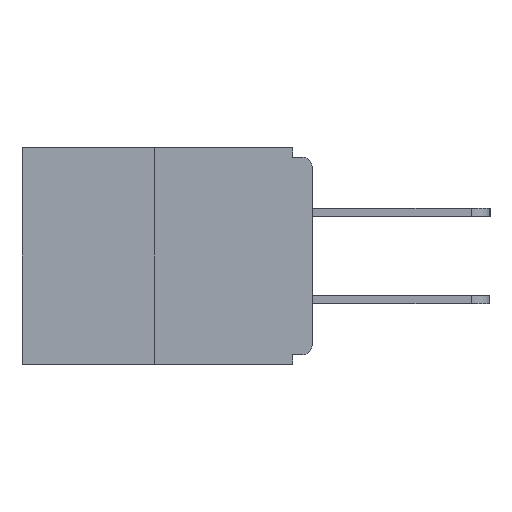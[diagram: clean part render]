
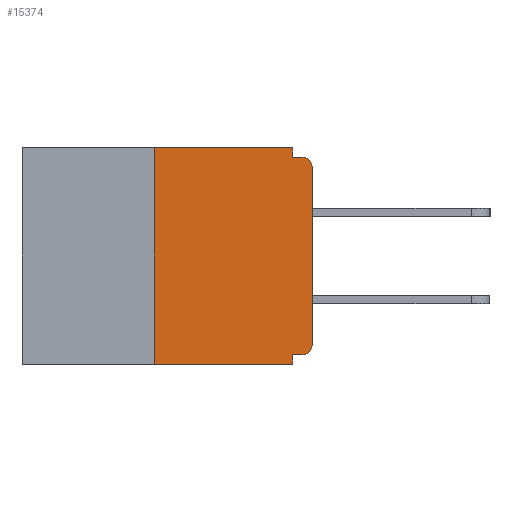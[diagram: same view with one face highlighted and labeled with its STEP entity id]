
A CAD part, left-side view. The second image highlights one B-rep face of the part: STEP entity #15374.
In plain terms, the highlighted planar face has unit normal (-1, 0, 0).
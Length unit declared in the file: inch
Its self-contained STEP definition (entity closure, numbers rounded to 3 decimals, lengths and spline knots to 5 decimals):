
#116 = ORIENTED_EDGE ( 'NONE', *, *, #5797, .F. ) ;
#548 = AXIS2_PLACEMENT_3D ( 'NONE', #4685, #12397, #15321 ) ;
#725 = VERTEX_POINT ( 'NONE', #12813 ) ;
#826 = ORIENTED_EDGE ( 'NONE', *, *, #8485, .T. ) ;
#909 = VECTOR ( 'NONE', #10721, 39.37008 ) ;
#1243 = EDGE_CURVE ( 'NONE', #17369, #4859, #12869, .T. ) ;
#1270 = DIRECTION ( 'NONE',  ( 0., 0., 1. ) ) ;
#1637 = LINE ( 'NONE', #8175, #12702 ) ;
#1675 = ORIENTED_EDGE ( 'NONE', *, *, #10460, .F. ) ;
#1790 = CIRCLE ( 'NONE', #548, 0.015 ) ;
#2052 = EDGE_CURVE ( 'NONE', #7994, #5197, #8822, .T. ) ;
#2444 = DIRECTION ( 'NONE',  ( 0., 0., -1. ) ) ;
#2753 = EDGE_CURVE ( 'NONE', #4544, #6234, #12340, .T. ) ;
#2941 = DIRECTION ( 'NONE',  ( 0., 1., 0. ) ) ;
#2968 = CARTESIAN_POINT ( 'NONE',  ( 0., 0.46, -0.343 ) ) ;
#3226 = VECTOR ( 'NONE', #10887, 39.37008 ) ;
#3380 = EDGE_CURVE ( 'NONE', #6234, #16784, #4997, .T. ) ;
#4280 = ORIENTED_EDGE ( 'NONE', *, *, #11982, .F. ) ;
#4544 = VERTEX_POINT ( 'NONE', #17344 ) ;
#4685 = CARTESIAN_POINT ( 'NONE',  ( 0., 0.015, -0.313 ) ) ;
#4764 = ORIENTED_EDGE ( 'NONE', *, *, #7035, .F. ) ;
#4859 = VERTEX_POINT ( 'NONE', #5698 ) ;
#4997 = CIRCLE ( 'NONE', #11948, 0.015 ) ;
#5197 = VERTEX_POINT ( 'NONE', #12374 ) ;
#5629 = EDGE_CURVE ( 'NONE', #18832, #5197, #1637, .T. ) ;
#5698 = CARTESIAN_POINT ( 'NONE',  ( 0., 0.031, -0.015 ) ) ;
#5797 = EDGE_CURVE ( 'NONE', #725, #17369, #9848, .T. ) ;
#6234 = VERTEX_POINT ( 'NONE', #7542 ) ;
#6397 = CARTESIAN_POINT ( 'NONE',  ( 0., 0.015, -0.03 ) ) ;
#7035 = EDGE_CURVE ( 'NONE', #7994, #725, #15952, .T. ) ;
#7080 = LINE ( 'NONE', #16276, #18006 ) ;
#7542 = CARTESIAN_POINT ( 'NONE',  ( 0., 0., -0.03 ) ) ;
#7641 = VECTOR ( 'NONE', #10596, 39.37008 ) ;
#7994 = VERTEX_POINT ( 'NONE', #11070 ) ;
#8175 = CARTESIAN_POINT ( 'NONE',  ( 0., 0.031, -0.343 ) ) ;
#8190 = EDGE_LOOP ( 'NONE', ( #116, #4764, #17671, #8336, #1675, #826, #17437, #17087, #4280, #19450 ) ) ;
#8336 = ORIENTED_EDGE ( 'NONE', *, *, #5629, .F. ) ;
#8485 = EDGE_CURVE ( 'NONE', #15748, #4544, #1790, .T. ) ;
#8822 = LINE ( 'NONE', #2968, #7641 ) ;
#9034 = VECTOR ( 'NONE', #15304, 39.37008 ) ;
#9529 = CARTESIAN_POINT ( 'NONE',  ( 0., 0.031, 0. ) ) ;
#9639 = CARTESIAN_POINT ( 'NONE',  ( 0., 0.015, -0.328 ) ) ;
#9848 = LINE ( 'NONE', #10450, #909 ) ;
#10426 = CARTESIAN_POINT ( 'NONE',  ( 0., 0., -0.328 ) ) ;
#10450 = CARTESIAN_POINT ( 'NONE',  ( 0., 0.46, 0. ) ) ;
#10460 = EDGE_CURVE ( 'NONE', #15748, #18832, #16341, .T. ) ;
#10596 = DIRECTION ( 'NONE',  ( 0., -1., 0. ) ) ;
#10721 = DIRECTION ( 'NONE',  ( 0., -1., 0. ) ) ;
#10887 = DIRECTION ( 'NONE',  ( 0., 0., -1. ) ) ;
#11070 = CARTESIAN_POINT ( 'NONE',  ( 0., 0.25, -0.343 ) ) ;
#11948 = AXIS2_PLACEMENT_3D ( 'NONE', #6397, #18716, #12524 ) ;
#11982 = EDGE_CURVE ( 'NONE', #4859, #16784, #7080, .T. ) ;
#12021 = DIRECTION ( 'NONE',  ( 0., -1., 0. ) ) ;
#12305 = DIRECTION ( 'NONE',  ( 1., 0., 0. ) ) ;
#12340 = LINE ( 'NONE', #18499, #9034 ) ;
#12374 = CARTESIAN_POINT ( 'NONE',  ( 0., 0.031, -0.343 ) ) ;
#12397 = DIRECTION ( 'NONE',  ( -1., 0., 0. ) ) ;
#12412 = CARTESIAN_POINT ( 'NONE',  ( 0., 0.031, 0. ) ) ;
#12524 = DIRECTION ( 'NONE',  ( 0., 0., -1. ) ) ;
#12702 = VECTOR ( 'NONE', #2444, 39.37008 ) ;
#12813 = CARTESIAN_POINT ( 'NONE',  ( 0., 0.25, 0. ) ) ;
#12869 = LINE ( 'NONE', #9529, #3226 ) ;
#13877 = CARTESIAN_POINT ( 'NONE',  ( 0., 0.031, -0.328 ) ) ;
#15304 = DIRECTION ( 'NONE',  ( 0., 0., 1. ) ) ;
#15321 = DIRECTION ( 'NONE',  ( 0., 0., -1. ) ) ;
#15374 = ADVANCED_FACE ( 'NONE', ( #17642 ), #16702, .F. ) ;
#15748 = VERTEX_POINT ( 'NONE', #9639 ) ;
#15952 = LINE ( 'NONE', #16166, #16171 ) ;
#16166 = CARTESIAN_POINT ( 'NONE',  ( 0., 0.25, 0. ) ) ;
#16171 = VECTOR ( 'NONE', #1270, 39.37008 ) ;
#16276 = CARTESIAN_POINT ( 'NONE',  ( 0., 0., -0.015 ) ) ;
#16341 = LINE ( 'NONE', #10426, #17104 ) ;
#16702 = PLANE ( 'NONE',  #17232 ) ;
#16784 = VERTEX_POINT ( 'NONE', #18428 ) ;
#16907 = CARTESIAN_POINT ( 'NONE',  ( 0., 0.46, 0. ) ) ;
#17087 = ORIENTED_EDGE ( 'NONE', *, *, #3380, .T. ) ;
#17104 = VECTOR ( 'NONE', #2941, 39.37008 ) ;
#17232 = AXIS2_PLACEMENT_3D ( 'NONE', #16907, #12305, #18367 ) ;
#17344 = CARTESIAN_POINT ( 'NONE',  ( 0., 0., -0.313 ) ) ;
#17369 = VERTEX_POINT ( 'NONE', #12412 ) ;
#17437 = ORIENTED_EDGE ( 'NONE', *, *, #2753, .T. ) ;
#17642 = FACE_OUTER_BOUND ( 'NONE', #8190, .T. ) ;
#17671 = ORIENTED_EDGE ( 'NONE', *, *, #2052, .T. ) ;
#18006 = VECTOR ( 'NONE', #12021, 39.37008 ) ;
#18367 = DIRECTION ( 'NONE',  ( 0., 0., -1. ) ) ;
#18428 = CARTESIAN_POINT ( 'NONE',  ( 0., 0.015, -0.015 ) ) ;
#18499 = CARTESIAN_POINT ( 'NONE',  ( 0., 0., 0. ) ) ;
#18716 = DIRECTION ( 'NONE',  ( -1., 0., 0. ) ) ;
#18832 = VERTEX_POINT ( 'NONE', #13877 ) ;
#19450 = ORIENTED_EDGE ( 'NONE', *, *, #1243, .F. ) ;
